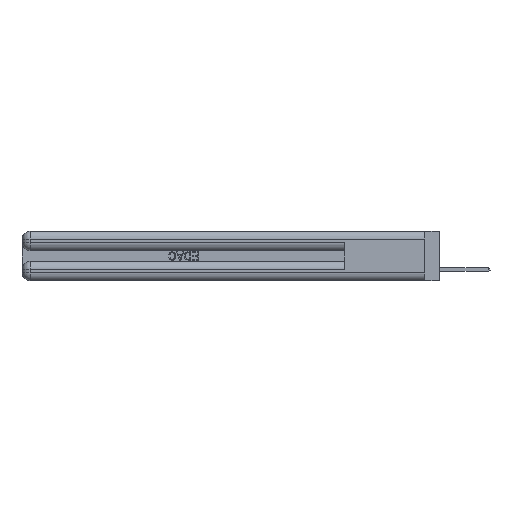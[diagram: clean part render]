
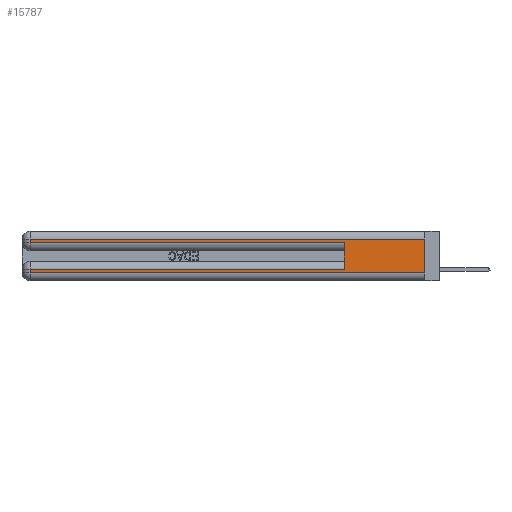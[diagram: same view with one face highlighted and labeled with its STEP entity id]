
A CAD part, left-side view. The second image highlights one B-rep face of the part: STEP entity #15787.
In plain terms, the highlighted planar face has unit normal (-1, 0, 0).
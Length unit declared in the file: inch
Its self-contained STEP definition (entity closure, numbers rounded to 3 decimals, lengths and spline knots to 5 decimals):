
#454 = CARTESIAN_POINT ( 'NONE',  ( 0., 2.94, 0.37 ) ) ;
#597 = EDGE_LOOP ( 'NONE', ( #25257, #19163, #17142, #5481, #27164, #33342, #12909, #18380 ) ) ;
#1068 = CARTESIAN_POINT ( 'NONE',  ( 0., 0., 0.37 ) ) ;
#1419 = CARTESIAN_POINT ( 'NONE',  ( 0., 0., 0.06 ) ) ;
#1604 = CARTESIAN_POINT ( 'NONE',  ( 0., 2.94, 0.37 ) ) ;
#1919 = DIRECTION ( 'NONE',  ( 0., -1., 0. ) ) ;
#2492 = LINE ( 'NONE', #6935, #33100 ) ;
#3893 = VECTOR ( 'NONE', #20376, 39.37008 ) ;
#3945 = EDGE_CURVE ( 'NONE', #44035, #12590, #38815, .T. ) ;
#4943 = EDGE_CURVE ( 'NONE', #12590, #22609, #26497, .T. ) ;
#5481 = ORIENTED_EDGE ( 'NONE', *, *, #31402, .T. ) ;
#6935 = CARTESIAN_POINT ( 'NONE',  ( 0., 0.6, 0.145 ) ) ;
#7910 = VERTEX_POINT ( 'NONE', #22299 ) ;
#8438 = FACE_OUTER_BOUND ( 'NONE', #597, .T. ) ;
#8648 = CARTESIAN_POINT ( 'NONE',  ( 0., 2.94, 0.06 ) ) ;
#10149 = CARTESIAN_POINT ( 'NONE',  ( 0., 0., 0.285 ) ) ;
#10414 = DIRECTION ( 'NONE',  ( 0., 0., -1. ) ) ;
#10754 = LINE ( 'NONE', #34767, #43012 ) ;
#10937 = EDGE_CURVE ( 'NONE', #24493, #40527, #36713, .T. ) ;
#11143 = VECTOR ( 'NONE', #1919, 39.37008 ) ;
#11403 = VERTEX_POINT ( 'NONE', #30999 ) ;
#11480 = VECTOR ( 'NONE', #14353, 39.37008 ) ;
#12590 = VERTEX_POINT ( 'NONE', #40277 ) ;
#12613 = LINE ( 'NONE', #16238, #24802 ) ;
#12909 = ORIENTED_EDGE ( 'NONE', *, *, #27817, .T. ) ;
#14353 = DIRECTION ( 'NONE',  ( 0., 0., -1. ) ) ;
#14397 = DIRECTION ( 'NONE',  ( 0., 0., 1. ) ) ;
#15436 = PLANE ( 'NONE',  #31013 ) ;
#15787 = ADVANCED_FACE ( 'NONE', ( #8438 ), #15436, .F. ) ;
#16238 = CARTESIAN_POINT ( 'NONE',  ( 0., 0., 0.085 ) ) ;
#16560 = VERTEX_POINT ( 'NONE', #32762 ) ;
#17142 = ORIENTED_EDGE ( 'NONE', *, *, #4943, .T. ) ;
#18380 = ORIENTED_EDGE ( 'NONE', *, *, #10937, .T. ) ;
#19163 = ORIENTED_EDGE ( 'NONE', *, *, #3945, .T. ) ;
#19296 = DIRECTION ( 'NONE',  ( 1., 0., 0. ) ) ;
#20338 = EDGE_CURVE ( 'NONE', #11403, #7910, #2492, .T. ) ;
#20376 = DIRECTION ( 'NONE',  ( 0., -1., 0. ) ) ;
#22299 = CARTESIAN_POINT ( 'NONE',  ( 0., 0.6, 0.285 ) ) ;
#22609 = VERTEX_POINT ( 'NONE', #26940 ) ;
#22888 = DIRECTION ( 'NONE',  ( 0., 0., -1. ) ) ;
#24471 = DIRECTION ( 'NONE',  ( 0., 1., 0. ) ) ;
#24493 = VERTEX_POINT ( 'NONE', #8648 ) ;
#24802 = VECTOR ( 'NONE', #40650, 39.37008 ) ;
#24821 = VECTOR ( 'NONE', #29922, 39.37008 ) ;
#25257 = ORIENTED_EDGE ( 'NONE', *, *, #35976, .F. ) ;
#26497 = LINE ( 'NONE', #1604, #24821 ) ;
#26940 = CARTESIAN_POINT ( 'NONE',  ( 0., 2.94, 0.285 ) ) ;
#27164 = ORIENTED_EDGE ( 'NONE', *, *, #20338, .F. ) ;
#27817 = EDGE_CURVE ( 'NONE', #16560, #24493, #33107, .T. ) ;
#29377 = VECTOR ( 'NONE', #24471, 39.37008 ) ;
#29922 = DIRECTION ( 'NONE',  ( 0., 0., -1. ) ) ;
#30090 = CARTESIAN_POINT ( 'NONE',  ( 0., 0., 0.06 ) ) ;
#30999 = CARTESIAN_POINT ( 'NONE',  ( 0., 0.6, 0.085 ) ) ;
#31013 = AXIS2_PLACEMENT_3D ( 'NONE', #1068, #19296, #22888 ) ;
#31402 = EDGE_CURVE ( 'NONE', #22609, #7910, #33383, .T. ) ;
#32762 = CARTESIAN_POINT ( 'NONE',  ( 0., 2.94, 0.085 ) ) ;
#33100 = VECTOR ( 'NONE', #14397, 39.37008 ) ;
#33107 = LINE ( 'NONE', #454, #11480 ) ;
#33342 = ORIENTED_EDGE ( 'NONE', *, *, #34144, .T. ) ;
#33383 = LINE ( 'NONE', #10149, #3893 ) ;
#34144 = EDGE_CURVE ( 'NONE', #11403, #16560, #12613, .T. ) ;
#34767 = CARTESIAN_POINT ( 'NONE',  ( 0., 0., 0.37 ) ) ;
#35027 = CARTESIAN_POINT ( 'NONE',  ( 0., 0., 0.31 ) ) ;
#35976 = EDGE_CURVE ( 'NONE', #44035, #40527, #10754, .T. ) ;
#36713 = LINE ( 'NONE', #30090, #11143 ) ;
#37565 = CARTESIAN_POINT ( 'NONE',  ( 0., 0., 0.31 ) ) ;
#38815 = LINE ( 'NONE', #35027, #29377 ) ;
#40277 = CARTESIAN_POINT ( 'NONE',  ( 0., 2.94, 0.31 ) ) ;
#40527 = VERTEX_POINT ( 'NONE', #1419 ) ;
#40650 = DIRECTION ( 'NONE',  ( 0., 1., 0. ) ) ;
#43012 = VECTOR ( 'NONE', #10414, 39.37008 ) ;
#44035 = VERTEX_POINT ( 'NONE', #37565 ) ;
